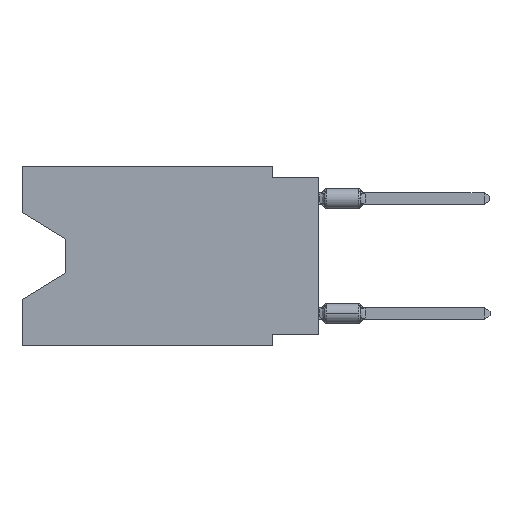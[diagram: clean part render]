
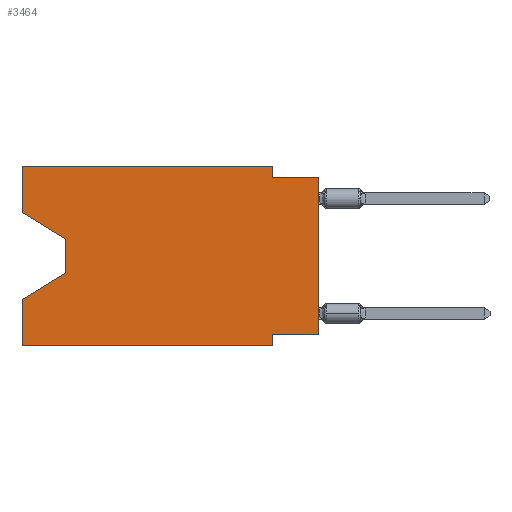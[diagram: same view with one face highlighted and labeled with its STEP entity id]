
A CAD part, left-side view. The second image highlights one B-rep face of the part: STEP entity #3464.
In plain terms, the highlighted planar face has unit normal (-1, 0, 0).
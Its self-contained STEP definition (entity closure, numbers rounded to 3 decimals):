
#503 = LINE ( 'NONE', #5469, #10576 ) ;
#778 = VECTOR ( 'NONE', #17096, 1000. ) ;
#1055 = CARTESIAN_POINT ( 'NONE',  ( 0., 16.383, -9.906 ) ) ;
#1227 = ORIENTED_EDGE ( 'NONE', *, *, #9730, .F. ) ;
#1301 = DIRECTION ( 'NONE',  ( 0., 0., -1. ) ) ;
#1337 = DIRECTION ( 'NONE',  ( 0., -0.855, -0.519 ) ) ;
#1481 = LINE ( 'NONE', #8071, #10292 ) ;
#1620 = VECTOR ( 'NONE', #1301, 1000. ) ;
#1900 = VECTOR ( 'NONE', #2713, 1000. ) ;
#1925 = CARTESIAN_POINT ( 'NONE',  ( 0., 16.383, -2.546 ) ) ;
#1960 = EDGE_CURVE ( 'NONE', #13272, #11355, #3361, .T. ) ;
#2044 = CARTESIAN_POINT ( 'NONE',  ( 0., 2.54, -0.635 ) ) ;
#2146 = ORIENTED_EDGE ( 'NONE', *, *, #3703, .F. ) ;
#2713 = DIRECTION ( 'NONE',  ( 0., 0., -1. ) ) ;
#2967 = CARTESIAN_POINT ( 'NONE',  ( 0., 16.383, -2.546 ) ) ;
#3361 = LINE ( 'NONE', #14608, #13525 ) ;
#3464 = ADVANCED_FACE ( 'NONE', ( #19676 ), #8302, .F. ) ;
#3671 = LINE ( 'NONE', #3982, #778 ) ;
#3703 = EDGE_CURVE ( 'NONE', #13272, #8237, #3671, .T. ) ;
#3982 = CARTESIAN_POINT ( 'NONE',  ( 0., 0., -9.271 ) ) ;
#4221 = CARTESIAN_POINT ( 'NONE',  ( 0., 13.97, -4.013 ) ) ;
#4352 = ORIENTED_EDGE ( 'NONE', *, *, #19072, .F. ) ;
#4513 = DIRECTION ( 'NONE',  ( 0., -1., 0. ) ) ;
#4654 = ORIENTED_EDGE ( 'NONE', *, *, #12143, .T. ) ;
#5469 = CARTESIAN_POINT ( 'NONE',  ( 0., 16.383, 0. ) ) ;
#5570 = CARTESIAN_POINT ( 'NONE',  ( 0., 2.54, 0. ) ) ;
#6155 = CARTESIAN_POINT ( 'NONE',  ( 0., 13.97, -4.013 ) ) ;
#6505 = VECTOR ( 'NONE', #9132, 1000. ) ;
#6968 = AXIS2_PLACEMENT_3D ( 'NONE', #7979, #19792, #16550 ) ;
#7033 = ORIENTED_EDGE ( 'NONE', *, *, #20622, .F. ) ;
#7354 = DIRECTION ( 'NONE',  ( 0., -1., 0. ) ) ;
#7542 = VECTOR ( 'NONE', #12181, 1000. ) ;
#7979 = CARTESIAN_POINT ( 'NONE',  ( 0., 16.383, 0. ) ) ;
#8071 = CARTESIAN_POINT ( 'NONE',  ( 0., 16.383, 0. ) ) ;
#8237 = VERTEX_POINT ( 'NONE', #16033 ) ;
#8302 = PLANE ( 'NONE',  #6968 ) ;
#8478 = CARTESIAN_POINT ( 'NONE',  ( 0., 0., -0.635 ) ) ;
#8510 = VERTEX_POINT ( 'NONE', #2044 ) ;
#8678 = CARTESIAN_POINT ( 'NONE',  ( 0., 13.97, -5.893 ) ) ;
#9132 = DIRECTION ( 'NONE',  ( 0., 0.855, -0.519 ) ) ;
#9198 = CARTESIAN_POINT ( 'NONE',  ( 0., 0., -0.635 ) ) ;
#9244 = CARTESIAN_POINT ( 'NONE',  ( 0., 13.97, -5.893 ) ) ;
#9283 = EDGE_CURVE ( 'NONE', #8510, #11355, #14397, .T. ) ;
#9342 = EDGE_CURVE ( 'NONE', #8237, #17000, #20798, .T. ) ;
#9612 = ORIENTED_EDGE ( 'NONE', *, *, #19177, .T. ) ;
#9626 = DIRECTION ( 'NONE',  ( 0., 0., 1. ) ) ;
#9730 = EDGE_CURVE ( 'NONE', #19012, #13032, #503, .T. ) ;
#10222 = DIRECTION ( 'NONE',  ( 0., -1., 0. ) ) ;
#10292 = VECTOR ( 'NONE', #21282, 1000. ) ;
#10576 = VECTOR ( 'NONE', #10222, 1000. ) ;
#10596 = VERTEX_POINT ( 'NONE', #18512 ) ;
#10935 = CARTESIAN_POINT ( 'NONE',  ( 0., 2.54, -9.906 ) ) ;
#11335 = ORIENTED_EDGE ( 'NONE', *, *, #9283, .F. ) ;
#11355 = VERTEX_POINT ( 'NONE', #8478 ) ;
#11446 = ORIENTED_EDGE ( 'NONE', *, *, #20752, .F. ) ;
#11703 = VECTOR ( 'NONE', #1337, 1000. ) ;
#11983 = LINE ( 'NONE', #15129, #14105 ) ;
#12113 = ORIENTED_EDGE ( 'NONE', *, *, #20894, .T. ) ;
#12143 = EDGE_CURVE ( 'NONE', #14457, #13995, #16355, .T. ) ;
#12181 = DIRECTION ( 'NONE',  ( 0., 0., -1. ) ) ;
#12465 = VERTEX_POINT ( 'NONE', #21366 ) ;
#13032 = VERTEX_POINT ( 'NONE', #16918 ) ;
#13262 = ORIENTED_EDGE ( 'NONE', *, *, #9342, .F. ) ;
#13272 = VERTEX_POINT ( 'NONE', #15454 ) ;
#13525 = VECTOR ( 'NONE', #9626, 1000. ) ;
#13806 = LINE ( 'NONE', #5570, #7542 ) ;
#13995 = VERTEX_POINT ( 'NONE', #8678 ) ;
#14105 = VECTOR ( 'NONE', #18603, 1000. ) ;
#14397 = LINE ( 'NONE', #9198, #20557 ) ;
#14457 = VERTEX_POINT ( 'NONE', #4221 ) ;
#14608 = CARTESIAN_POINT ( 'NONE',  ( 0., 0., 0. ) ) ;
#15056 = EDGE_CURVE ( 'NONE', #17930, #14457, #17906, .T. ) ;
#15129 = CARTESIAN_POINT ( 'NONE',  ( 0., 16.383, 0. ) ) ;
#15454 = CARTESIAN_POINT ( 'NONE',  ( 0., 0., -9.271 ) ) ;
#15915 = CARTESIAN_POINT ( 'NONE',  ( 0., 2.54, -9.906 ) ) ;
#16033 = CARTESIAN_POINT ( 'NONE',  ( 0., 2.54, -9.271 ) ) ;
#16355 = LINE ( 'NONE', #6155, #1620 ) ;
#16550 = DIRECTION ( 'NONE',  ( 0., 0., -1. ) ) ;
#16918 = CARTESIAN_POINT ( 'NONE',  ( 0., 2.54, 0. ) ) ;
#17000 = VERTEX_POINT ( 'NONE', #15915 ) ;
#17096 = DIRECTION ( 'NONE',  ( 0., 1., 0. ) ) ;
#17906 = LINE ( 'NONE', #2967, #11703 ) ;
#17930 = VERTEX_POINT ( 'NONE', #1925 ) ;
#18485 = ORIENTED_EDGE ( 'NONE', *, *, #15056, .T. ) ;
#18512 = CARTESIAN_POINT ( 'NONE',  ( 0., 16.383, -7.36 ) ) ;
#18572 = EDGE_LOOP ( 'NONE', ( #18485, #4654, #12113, #4352, #9612, #13262, #2146, #20391, #11335, #11446, #1227, #7033 ) ) ;
#18603 = DIRECTION ( 'NONE',  ( 0., 0., 1. ) ) ;
#18703 = CARTESIAN_POINT ( 'NONE',  ( 0., 16.383, 0. ) ) ;
#19012 = VERTEX_POINT ( 'NONE', #18703 ) ;
#19072 = EDGE_CURVE ( 'NONE', #12465, #10596, #11983, .T. ) ;
#19177 = EDGE_CURVE ( 'NONE', #12465, #17000, #19234, .T. ) ;
#19234 = LINE ( 'NONE', #1055, #19633 ) ;
#19316 = LINE ( 'NONE', #9244, #6505 ) ;
#19633 = VECTOR ( 'NONE', #4513, 1000. ) ;
#19676 = FACE_OUTER_BOUND ( 'NONE', #18572, .T. ) ;
#19792 = DIRECTION ( 'NONE',  ( 1., 0., 0. ) ) ;
#20391 = ORIENTED_EDGE ( 'NONE', *, *, #1960, .T. ) ;
#20557 = VECTOR ( 'NONE', #7354, 1000. ) ;
#20622 = EDGE_CURVE ( 'NONE', #17930, #19012, #1481, .T. ) ;
#20752 = EDGE_CURVE ( 'NONE', #13032, #8510, #13806, .T. ) ;
#20798 = LINE ( 'NONE', #10935, #1900 ) ;
#20894 = EDGE_CURVE ( 'NONE', #13995, #10596, #19316, .T. ) ;
#21282 = DIRECTION ( 'NONE',  ( 0., 0., 1. ) ) ;
#21366 = CARTESIAN_POINT ( 'NONE',  ( 0., 16.383, -9.906 ) ) ;
